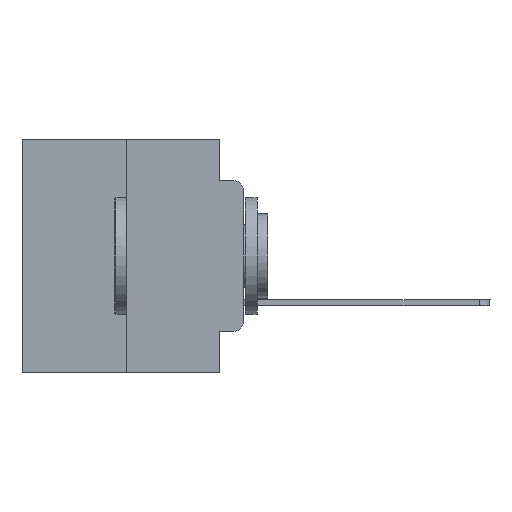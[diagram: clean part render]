
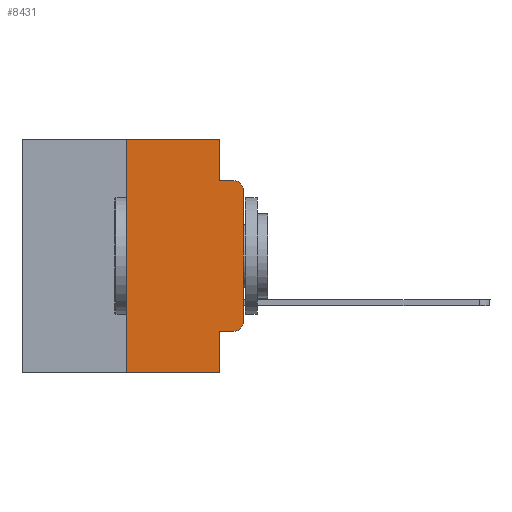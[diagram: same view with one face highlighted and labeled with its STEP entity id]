
A CAD part, left-side view. The second image highlights one B-rep face of the part: STEP entity #8431.
In plain terms, the highlighted planar face has unit normal (-1, 0, 0).
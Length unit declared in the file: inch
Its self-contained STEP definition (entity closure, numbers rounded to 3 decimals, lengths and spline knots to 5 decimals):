
#63 = EDGE_CURVE ( 'NONE', #13116, #24539, #20789, .T. ) ;
#177 = CARTESIAN_POINT ( 'NONE',  ( 0., 0.051, -0.0885 ) ) ;
#477 = EDGE_CURVE ( 'NONE', #22970, #15411, #2074, .T. ) ;
#799 = CARTESIAN_POINT ( 'NONE',  ( 0., 0.25, 0. ) ) ;
#1050 = CARTESIAN_POINT ( 'NONE',  ( 0., 0.051, -0.0885 ) ) ;
#1167 = VERTEX_POINT ( 'NONE', #4199 ) ;
#1458 = EDGE_CURVE ( 'NONE', #19850, #18319, #25926, .T. ) ;
#1857 = CARTESIAN_POINT ( 'NONE',  ( 0., 0.473, 0. ) ) ;
#1982 = DIRECTION ( 'NONE',  ( 0., -1., 0. ) ) ;
#2057 = DIRECTION ( 'NONE',  ( 0., -1., 0. ) ) ;
#2074 = LINE ( 'NONE', #799, #16582 ) ;
#2252 = EDGE_CURVE ( 'NONE', #1167, #24539, #10035, .T. ) ;
#2651 = EDGE_LOOP ( 'NONE', ( #21585, #15151, #19355, #4195, #21631, #12325, #17019, #24662, #8661, #26119 ) ) ;
#3307 = VECTOR ( 'NONE', #2057, 39.37008 ) ;
#3352 = FACE_OUTER_BOUND ( 'NONE', #2651, .T. ) ;
#3581 = EDGE_CURVE ( 'NONE', #8702, #13116, #20269, .T. ) ;
#4195 = ORIENTED_EDGE ( 'NONE', *, *, #3581, .F. ) ;
#4199 = CARTESIAN_POINT ( 'NONE',  ( 0., 0., -0.1085 ) ) ;
#5250 = DIRECTION ( 'NONE',  ( 0., -1., 0. ) ) ;
#6143 = VECTOR ( 'NONE', #5250, 39.37008 ) ;
#6268 = VECTOR ( 'NONE', #1982, 39.37008 ) ;
#7321 = CARTESIAN_POINT ( 'NONE',  ( 0., 0.02, -0.1085 ) ) ;
#7741 = DIRECTION ( 'NONE',  ( -1., 0., 0. ) ) ;
#7807 = DIRECTION ( 'NONE',  ( 0., 0., -1. ) ) ;
#8431 = ADVANCED_FACE ( 'NONE', ( #3352 ), #14207, .F. ) ;
#8661 = ORIENTED_EDGE ( 'NONE', *, *, #16342, .T. ) ;
#8702 = VERTEX_POINT ( 'NONE', #8867 ) ;
#8867 = CARTESIAN_POINT ( 'NONE',  ( 0., 0.051, 0. ) ) ;
#9085 = VECTOR ( 'NONE', #17373, 39.37008 ) ;
#9326 = EDGE_CURVE ( 'NONE', #15411, #8702, #11674, .T. ) ;
#9715 = CARTESIAN_POINT ( 'NONE',  ( 0., 0.051, 0. ) ) ;
#10035 = CIRCLE ( 'NONE', #12649, 0.02 ) ;
#10036 = EDGE_CURVE ( 'NONE', #22126, #1167, #24280, .T. ) ;
#10689 = CARTESIAN_POINT ( 'NONE',  ( 0., 0.25, -0.5 ) ) ;
#10888 = AXIS2_PLACEMENT_3D ( 'NONE', #20000, #7741, #11704 ) ;
#11674 = LINE ( 'NONE', #14225, #3307 ) ;
#11704 = DIRECTION ( 'NONE',  ( 0., 0., -1. ) ) ;
#11922 = LINE ( 'NONE', #23692, #6143 ) ;
#12086 = CARTESIAN_POINT ( 'NONE',  ( 0., 0.25, 0. ) ) ;
#12325 = ORIENTED_EDGE ( 'NONE', *, *, #477, .F. ) ;
#12649 = AXIS2_PLACEMENT_3D ( 'NONE', #7321, #17970, #15898 ) ;
#13116 = VERTEX_POINT ( 'NONE', #1050 ) ;
#14188 = CARTESIAN_POINT ( 'NONE',  ( 0., 0.051, -0.4115 ) ) ;
#14207 = PLANE ( 'NONE',  #26470 ) ;
#14224 = CARTESIAN_POINT ( 'NONE',  ( 0., 0.02, -0.0885 ) ) ;
#14225 = CARTESIAN_POINT ( 'NONE',  ( 0., 0.473, 0. ) ) ;
#15074 = CARTESIAN_POINT ( 'NONE',  ( 0., 0.051, -0.5 ) ) ;
#15151 = ORIENTED_EDGE ( 'NONE', *, *, #2252, .T. ) ;
#15411 = VERTEX_POINT ( 'NONE', #12086 ) ;
#15519 = EDGE_CURVE ( 'NONE', #25916, #22126, #22984, .T. ) ;
#15557 = VECTOR ( 'NONE', #23379, 39.37008 ) ;
#15898 = DIRECTION ( 'NONE',  ( 0., 0., -1. ) ) ;
#16342 = EDGE_CURVE ( 'NONE', #19850, #25916, #11922, .T. ) ;
#16524 = CARTESIAN_POINT ( 'NONE',  ( 0., 0., -0.3915 ) ) ;
#16582 = VECTOR ( 'NONE', #24382, 39.37008 ) ;
#17019 = ORIENTED_EDGE ( 'NONE', *, *, #26640, .T. ) ;
#17373 = DIRECTION ( 'NONE',  ( 0., 0., 1. ) ) ;
#17745 = CARTESIAN_POINT ( 'NONE',  ( 0., 0.473, -0.5 ) ) ;
#17970 = DIRECTION ( 'NONE',  ( -1., 0., 0. ) ) ;
#18155 = VECTOR ( 'NONE', #23656, 39.37008 ) ;
#18319 = VERTEX_POINT ( 'NONE', #15074 ) ;
#18357 = DIRECTION ( 'NONE',  ( 1., 0., 0. ) ) ;
#19291 = VECTOR ( 'NONE', #7807, 39.37008 ) ;
#19355 = ORIENTED_EDGE ( 'NONE', *, *, #63, .F. ) ;
#19850 = VERTEX_POINT ( 'NONE', #14188 ) ;
#20000 = CARTESIAN_POINT ( 'NONE',  ( 0., 0.02, -0.3915 ) ) ;
#20269 = LINE ( 'NONE', #9715, #19291 ) ;
#20789 = LINE ( 'NONE', #177, #6268 ) ;
#21585 = ORIENTED_EDGE ( 'NONE', *, *, #10036, .T. ) ;
#21631 = ORIENTED_EDGE ( 'NONE', *, *, #9326, .F. ) ;
#21817 = CARTESIAN_POINT ( 'NONE',  ( 0., 0., 0. ) ) ;
#22055 = LINE ( 'NONE', #17745, #18155 ) ;
#22126 = VERTEX_POINT ( 'NONE', #16524 ) ;
#22525 = DIRECTION ( 'NONE',  ( 0., 0., -1. ) ) ;
#22970 = VERTEX_POINT ( 'NONE', #10689 ) ;
#22984 = CIRCLE ( 'NONE', #10888, 0.02 ) ;
#23379 = DIRECTION ( 'NONE',  ( 0., 0., -1. ) ) ;
#23656 = DIRECTION ( 'NONE',  ( 0., -1., 0. ) ) ;
#23692 = CARTESIAN_POINT ( 'NONE',  ( 0., 0.051, -0.4115 ) ) ;
#24280 = LINE ( 'NONE', #21817, #9085 ) ;
#24382 = DIRECTION ( 'NONE',  ( 0., 0., 1. ) ) ;
#24539 = VERTEX_POINT ( 'NONE', #14224 ) ;
#24662 = ORIENTED_EDGE ( 'NONE', *, *, #1458, .F. ) ;
#25391 = CARTESIAN_POINT ( 'NONE',  ( 0., 0.02, -0.4115 ) ) ;
#25541 = CARTESIAN_POINT ( 'NONE',  ( 0., 0.051, 0. ) ) ;
#25916 = VERTEX_POINT ( 'NONE', #25391 ) ;
#25926 = LINE ( 'NONE', #25541, #15557 ) ;
#26119 = ORIENTED_EDGE ( 'NONE', *, *, #15519, .T. ) ;
#26470 = AXIS2_PLACEMENT_3D ( 'NONE', #1857, #18357, #22525 ) ;
#26640 = EDGE_CURVE ( 'NONE', #22970, #18319, #22055, .T. ) ;
